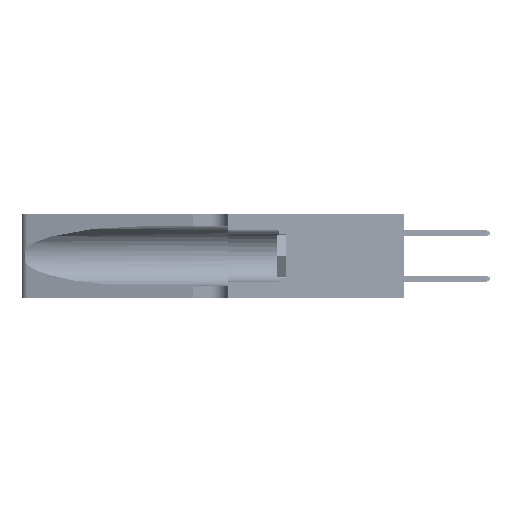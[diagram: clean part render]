
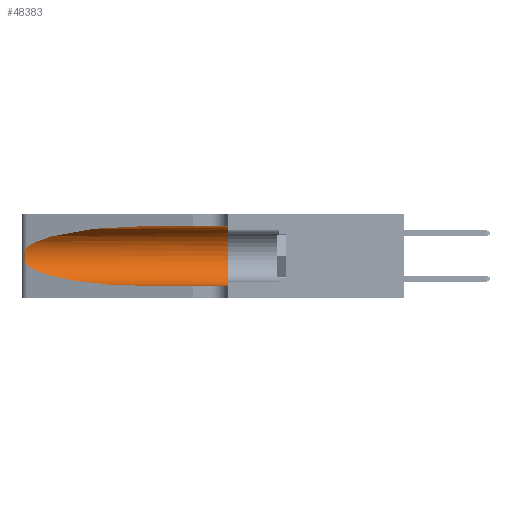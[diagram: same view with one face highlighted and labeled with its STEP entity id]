
A CAD part, left-side view. The second image highlights one B-rep face of the part: STEP entity #48383.
In plain terms, the highlighted cylindrical face has radius 3.308 mm (diameter 6.617 mm), a partial arc.
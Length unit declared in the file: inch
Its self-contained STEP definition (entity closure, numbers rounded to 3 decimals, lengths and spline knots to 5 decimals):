
#441 = FACE_OUTER_BOUND ( 'NONE', #28494, .T. ) ;
#1128 = CARTESIAN_POINT ( 'NONE',  ( 0.25787, 1.23484, 0.2124 ) ) ;
#2703 = VERTEX_POINT ( 'NONE', #26301 ) ;
#5310 = CARTESIAN_POINT ( 'NONE',  ( 0.26018, 1.23835, 0.19895 ) ) ;
#5314 = CARTESIAN_POINT ( 'NONE',  ( 0.2373, 1.15595, 0.08982 ) ) ;
#5631 = B_SPLINE_CURVE_WITH_KNOTS ( 'NONE', 3,
 ( #49987, #21568, #25672, #1128, #29758, #5310, #33851, #9442, #37915, #13541, #41988, #17673, #46099, #21746 ),
 .UNSPECIFIED., .F., .F.,
 ( 4, 2, 2, 2, 2, 2, 4 ),
 ( 0., 0.00027, 0.00053, 0.00107, 0.0016, 0.00187, 0.00214 ),
 .UNSPECIFIED. ) ;
#6829 = DIRECTION ( 'NONE',  ( 0., 0., -1. ) ) ;
#7398 = LINE ( 'NONE', #46699, #38607 ) ;
#7531 = CIRCLE ( 'NONE', #18456, 0.13025 ) ;
#9442 = CARTESIAN_POINT ( 'NONE',  ( 0.26075, 1.23896, 0.178 ) ) ;
#10950 = CARTESIAN_POINT ( 'NONE',  ( 0.1305, 0.35, 0.31525 ) ) ;
#11243 = ORIENTED_EDGE ( 'NONE', *, *, #26528, .T. ) ;
#12057 = VECTOR ( 'NONE', #35350, 39.37008 ) ;
#13541 = CARTESIAN_POINT ( 'NONE',  ( 0.25856, 1.23593, 0.16098 ) ) ;
#13833 = DIRECTION ( 'NONE',  ( 0., 1., 0. ) ) ;
#17558 = CARTESIAN_POINT ( 'NONE',  ( 0.2373, 1.15595, 0.28018 ) ) ;
#17673 = CARTESIAN_POINT ( 'NONE',  ( 0.25639, 1.23186, 0.15144 ) ) ;
#17676 = CARTESIAN_POINT ( 'NONE',  ( 0.18966, 0.96281, 0.05475 ) ) ;
#17903 = VERTEX_POINT ( 'NONE', #32003 ) ;
#18456 = AXIS2_PLACEMENT_3D ( 'NONE', #38185, #13833, #42273 ) ;
#19719 = CYLINDRICAL_SURFACE ( 'NONE', #23556, 0.13025 ) ;
#20357 = EDGE_CURVE ( 'NONE', #17903, #25580, #24201, .T. ) ;
#21568 = CARTESIAN_POINT ( 'NONE',  ( 0.25555, 1.22994, 0.2215 ) ) ;
#21735 = VERTEX_POINT ( 'NONE', #40185 ) ;
#21746 = CARTESIAN_POINT ( 'NONE',  ( 0.25487, 1.22718, 0.14631 ) ) ;
#23556 = AXIS2_PLACEMENT_3D ( 'NONE', #52386, #23998, #6829 ) ;
#23998 = DIRECTION ( 'NONE',  ( 0., -1., 0. ) ) ;
#24201 = LINE ( 'NONE', #31262, #12057 ) ;
#24635 =( BOUNDED_CURVE ( )  B_SPLINE_CURVE ( 3, ( #33854, #5314, #17676, #46104 ),
 .UNSPECIFIED., .F., .T. ) 
 B_SPLINE_CURVE_WITH_KNOTS ( ( 4, 4 ),
 ( 3.44316, 4.71239 ),
 .UNSPECIFIED. ) 
 CURVE ( )  GEOMETRIC_REPRESENTATION_ITEM ( )  RATIONAL_B_SPLINE_CURVE ( ( 1., 0.87, 0.87, 1. ) ) 
 REPRESENTATION_ITEM ( '' )  );
#25124 = ORIENTED_EDGE ( 'NONE', *, *, #25320, .F. ) ;
#25320 = EDGE_CURVE ( 'NONE', #25580, #44059, #7531, .T. ) ;
#25580 = VERTEX_POINT ( 'NONE', #10950 ) ;
#25672 = CARTESIAN_POINT ( 'NONE',  ( 0.25639, 1.23184, 0.21858 ) ) ;
#26301 = CARTESIAN_POINT ( 'NONE',  ( 0.1305, 0.72297, 0.05475 ) ) ;
#26452 = DIRECTION ( 'NONE',  ( 0., -1., 0. ) ) ;
#26528 = EDGE_CURVE ( 'NONE', #40840, #2703, #24635, .T. ) ;
#27191 = ORIENTED_EDGE ( 'NONE', *, *, #44858, .T. ) ;
#27826 = ORIENTED_EDGE ( 'NONE', *, *, #39476, .T. ) ;
#28485 = ORIENTED_EDGE ( 'NONE', *, *, #50048, .T. ) ;
#28494 = EDGE_LOOP ( 'NONE', ( #28485, #27191, #11243, #27826, #25124, #37807 ) ) ;
#29758 = CARTESIAN_POINT ( 'NONE',  ( 0.25854, 1.2359, 0.20912 ) ) ;
#30160 =( BOUNDED_CURVE ( )  B_SPLINE_CURVE ( 3, ( #37803, #41873, #17558, #45983 ),
 .UNSPECIFIED., .F., .F. ) 
 B_SPLINE_CURVE_WITH_KNOTS ( ( 4, 4 ),
 ( 1.5708, 2.84003 ),
 .UNSPECIFIED. ) 
 CURVE ( )  GEOMETRIC_REPRESENTATION_ITEM ( )  RATIONAL_B_SPLINE_CURVE ( ( 1., 0.87, 0.87, 1. ) ) 
 REPRESENTATION_ITEM ( '' )  );
#31262 = CARTESIAN_POINT ( 'NONE',  ( 0.1305, 1.61858, 0.31525 ) ) ;
#32003 = CARTESIAN_POINT ( 'NONE',  ( 0.1305, 0.72297, 0.31525 ) ) ;
#33851 = CARTESIAN_POINT ( 'NONE',  ( 0.26075, 1.23896, 0.19203 ) ) ;
#33854 = CARTESIAN_POINT ( 'NONE',  ( 0.25487, 1.22718, 0.14631 ) ) ;
#35350 = DIRECTION ( 'NONE',  ( 0., -1., 0. ) ) ;
#37803 = CARTESIAN_POINT ( 'NONE',  ( 0.1305, 0.72297, 0.31525 ) ) ;
#37807 = ORIENTED_EDGE ( 'NONE', *, *, #20357, .F. ) ;
#37915 = CARTESIAN_POINT ( 'NONE',  ( 0.26017, 1.23833, 0.17102 ) ) ;
#38185 = CARTESIAN_POINT ( 'NONE',  ( 0.1305, 0.35, 0.185 ) ) ;
#38607 = VECTOR ( 'NONE', #26452, 39.37008 ) ;
#39476 = EDGE_CURVE ( 'NONE', #2703, #44059, #7398, .T. ) ;
#40185 = CARTESIAN_POINT ( 'NONE',  ( 0.25487, 1.22718, 0.22369 ) ) ;
#40840 = VERTEX_POINT ( 'NONE', #47583 ) ;
#41176 = CARTESIAN_POINT ( 'NONE',  ( 0.1305, 0.35, 0.05475 ) ) ;
#41873 = CARTESIAN_POINT ( 'NONE',  ( 0.18966, 0.96281, 0.31525 ) ) ;
#41988 = CARTESIAN_POINT ( 'NONE',  ( 0.25789, 1.23486, 0.15765 ) ) ;
#42273 = DIRECTION ( 'NONE',  ( 0., 0., 1. ) ) ;
#44059 = VERTEX_POINT ( 'NONE', #41176 ) ;
#44858 = EDGE_CURVE ( 'NONE', #21735, #40840, #5631, .T. ) ;
#45983 = CARTESIAN_POINT ( 'NONE',  ( 0.25487, 1.22718, 0.22369 ) ) ;
#46099 = CARTESIAN_POINT ( 'NONE',  ( 0.25555, 1.22993, 0.14849 ) ) ;
#46104 = CARTESIAN_POINT ( 'NONE',  ( 0.1305, 0.72297, 0.05475 ) ) ;
#46699 = CARTESIAN_POINT ( 'NONE',  ( 0.1305, 1.61858, 0.05475 ) ) ;
#47583 = CARTESIAN_POINT ( 'NONE',  ( 0.25487, 1.22718, 0.14631 ) ) ;
#48383 = ADVANCED_FACE ( 'NONE', ( #441 ), #19719, .F. ) ;
#49987 = CARTESIAN_POINT ( 'NONE',  ( 0.25487, 1.22718, 0.22369 ) ) ;
#50048 = EDGE_CURVE ( 'NONE', #17903, #21735, #30160, .T. ) ;
#52386 = CARTESIAN_POINT ( 'NONE',  ( 0.1305, 1.61858, 0.185 ) ) ;
